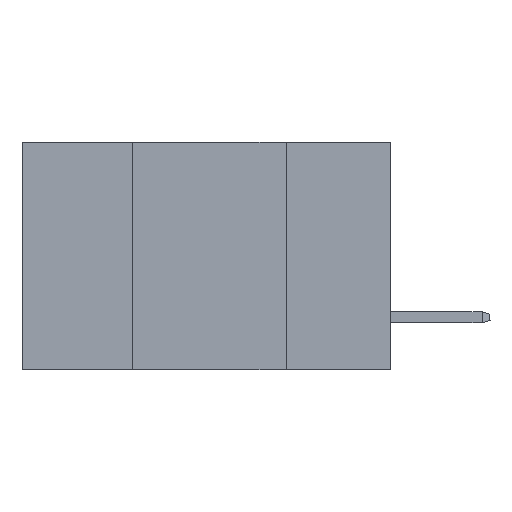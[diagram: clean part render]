
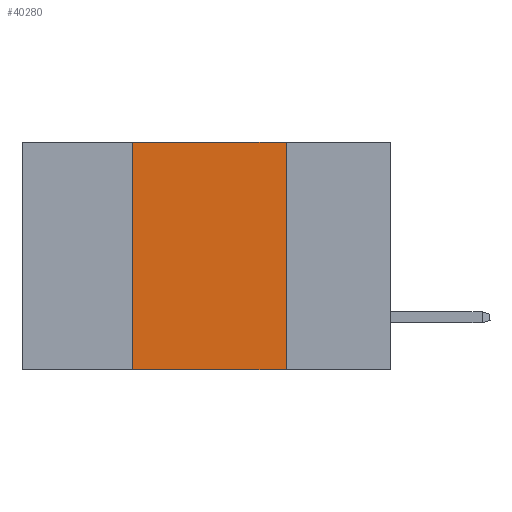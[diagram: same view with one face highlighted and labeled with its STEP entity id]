
A CAD part, left-side view. The second image highlights one B-rep face of the part: STEP entity #40280.
In plain terms, the highlighted planar face has unit normal (-1, 0, 0).
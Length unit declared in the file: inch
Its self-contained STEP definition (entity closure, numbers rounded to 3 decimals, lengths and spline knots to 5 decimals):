
#359 = CARTESIAN_POINT ( 'NONE',  ( 0., 0.17, -0.37 ) ) ;
#413 = CARTESIAN_POINT ( 'NONE',  ( 0., 0.42, 0. ) ) ;
#3842 = EDGE_CURVE ( 'NONE', #18429, #18136, #33043, .T. ) ;
#6549 = CARTESIAN_POINT ( 'NONE',  ( 0., 0.42, -0.37 ) ) ;
#6691 = EDGE_CURVE ( 'NONE', #18136, #14793, #38432, .T. ) ;
#6747 = ORIENTED_EDGE ( 'NONE', *, *, #19742, .F. ) ;
#7187 = VECTOR ( 'NONE', #27930, 39.37008 ) ;
#10075 = LINE ( 'NONE', #13592, #7187 ) ;
#10671 = VECTOR ( 'NONE', #24094, 39.37008 ) ;
#11302 = CARTESIAN_POINT ( 'NONE',  ( 0., 0.42, 0. ) ) ;
#13592 = CARTESIAN_POINT ( 'NONE',  ( 0., 0.17, 0. ) ) ;
#14397 = CARTESIAN_POINT ( 'NONE',  ( 0., 0.6, 0. ) ) ;
#14793 = VERTEX_POINT ( 'NONE', #41064 ) ;
#14871 = PLANE ( 'NONE',  #42120 ) ;
#17940 = DIRECTION ( 'NONE',  ( 1., 0., 0. ) ) ;
#18035 = DIRECTION ( 'NONE',  ( 0., 0., 1. ) ) ;
#18136 = VERTEX_POINT ( 'NONE', #11302 ) ;
#18429 = VERTEX_POINT ( 'NONE', #6549 ) ;
#19717 = VECTOR ( 'NONE', #41771, 39.37008 ) ;
#19742 = EDGE_CURVE ( 'NONE', #14793, #36079, #10075, .T. ) ;
#21800 = ORIENTED_EDGE ( 'NONE', *, *, #3842, .F. ) ;
#24094 = DIRECTION ( 'NONE',  ( 0., -1., 0. ) ) ;
#26089 = ORIENTED_EDGE ( 'NONE', *, *, #41876, .T. ) ;
#26652 = ORIENTED_EDGE ( 'NONE', *, *, #6691, .F. ) ;
#27930 = DIRECTION ( 'NONE',  ( 0., 0., -1. ) ) ;
#28736 = DIRECTION ( 'NONE',  ( 0., 0., -1. ) ) ;
#31366 = CARTESIAN_POINT ( 'NONE',  ( 0., 0.6, 0. ) ) ;
#31402 = LINE ( 'NONE', #34468, #19717 ) ;
#33043 = LINE ( 'NONE', #413, #44729 ) ;
#34468 = CARTESIAN_POINT ( 'NONE',  ( 0., 0.6, -0.37 ) ) ;
#36079 = VERTEX_POINT ( 'NONE', #359 ) ;
#38432 = LINE ( 'NONE', #31366, #10671 ) ;
#40258 = FACE_OUTER_BOUND ( 'NONE', #42812, .T. ) ;
#40280 = ADVANCED_FACE ( 'NONE', ( #40258 ), #14871, .F. ) ;
#41064 = CARTESIAN_POINT ( 'NONE',  ( 0., 0.17, 0. ) ) ;
#41771 = DIRECTION ( 'NONE',  ( 0., -1., 0. ) ) ;
#41876 = EDGE_CURVE ( 'NONE', #18429, #36079, #31402, .T. ) ;
#42120 = AXIS2_PLACEMENT_3D ( 'NONE', #14397, #17940, #28736 ) ;
#42812 = EDGE_LOOP ( 'NONE', ( #6747, #26652, #21800, #26089 ) ) ;
#44729 = VECTOR ( 'NONE', #18035, 39.37008 ) ;
